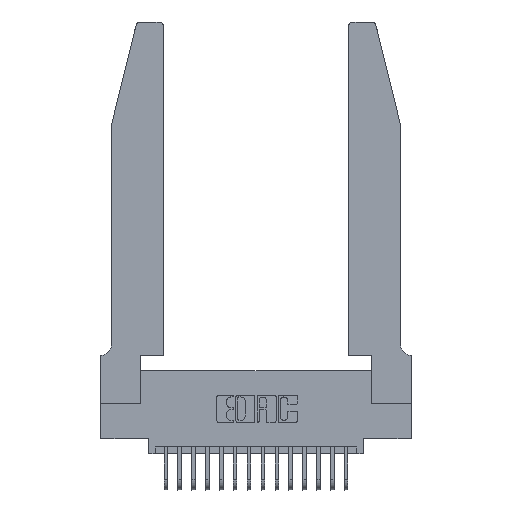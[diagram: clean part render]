
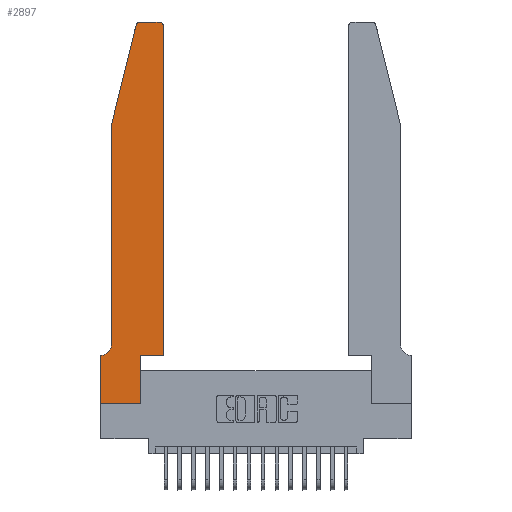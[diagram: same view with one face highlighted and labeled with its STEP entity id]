
A CAD part, top view. The second image highlights one B-rep face of the part: STEP entity #2897.
In plain terms, the highlighted planar face has unit normal (0, 0, 1).
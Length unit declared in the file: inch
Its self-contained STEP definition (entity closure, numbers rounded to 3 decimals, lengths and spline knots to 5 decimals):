
#325 = DIRECTION ( 'NONE',  ( -0.239, -0.971, 0. ) ) ;
#624 = DIRECTION ( 'NONE',  ( 0., 1., 0. ) ) ;
#640 = DIRECTION ( 'NONE',  ( 1., 0., 0. ) ) ;
#655 = VECTOR ( 'NONE', #14205, 39.37008 ) ;
#706 = EDGE_CURVE ( 'NONE', #8386, #5808, #14418, .T. ) ;
#888 = DIRECTION ( 'NONE',  ( 0., 0., 1. ) ) ;
#903 = ORIENTED_EDGE ( 'NONE', *, *, #10940, .T. ) ;
#1069 = LINE ( 'NONE', #20394, #10532 ) ;
#1198 = VERTEX_POINT ( 'NONE', #11049 ) ;
#1273 = DIRECTION ( 'NONE',  ( 0., 0., 1. ) ) ;
#1739 = DIRECTION ( 'NONE',  ( 0., 0., -1. ) ) ;
#1760 = VECTOR ( 'NONE', #624, 39.37008 ) ;
#2020 = CARTESIAN_POINT ( 'NONE',  ( 0.0755, 2., 0.37 ) ) ;
#2358 = VERTEX_POINT ( 'NONE', #17451 ) ;
#2367 = DIRECTION ( 'NONE',  ( 1., 0., 0. ) ) ;
#2600 = CARTESIAN_POINT ( 'NONE',  ( 0.4505, 0.35, 0.37 ) ) ;
#2601 = VECTOR ( 'NONE', #11731, 39.37008 ) ;
#2897 = ADVANCED_FACE ( 'NONE', ( #16101 ), #9296, .T. ) ;
#2921 = CARTESIAN_POINT ( 'NONE',  ( 0.284, 2.72, 0.37 ) ) ;
#3014 = CARTESIAN_POINT ( 'NONE',  ( 0.2865, 0.35, 0.37 ) ) ;
#3287 = CARTESIAN_POINT ( 'NONE',  ( 0.0755, 0.42, 0.37 ) ) ;
#3409 = CARTESIAN_POINT ( 'NONE',  ( 0.4205, 2.72, 0.37 ) ) ;
#3620 = VERTEX_POINT ( 'NONE', #20983 ) ;
#3639 = ORIENTED_EDGE ( 'NONE', *, *, #14645, .T. ) ;
#3955 = CARTESIAN_POINT ( 'NONE',  ( 0., 0., 0.37 ) ) ;
#4011 = EDGE_CURVE ( 'NONE', #3620, #1198, #1069, .T. ) ;
#4098 = ORIENTED_EDGE ( 'NONE', *, *, #18431, .T. ) ;
#4286 = EDGE_CURVE ( 'NONE', #17471, #16448, #14063, .T. ) ;
#4287 = CARTESIAN_POINT ( 'NONE',  ( 0.2865, 0., 0.37 ) ) ;
#4848 = VERTEX_POINT ( 'NONE', #5759 ) ;
#4916 = VECTOR ( 'NONE', #325, 39.37008 ) ;
#5116 = VERTEX_POINT ( 'NONE', #19408 ) ;
#5130 = DIRECTION ( 'NONE',  ( 1., 0., 0. ) ) ;
#5552 = LINE ( 'NONE', #20223, #8934 ) ;
#5682 = CARTESIAN_POINT ( 'NONE',  ( 0.2865, 0.35, 0.37 ) ) ;
#5715 = CARTESIAN_POINT ( 'NONE',  ( 0., 0., 0.37 ) ) ;
#5719 = AXIS2_PLACEMENT_3D ( 'NONE', #11769, #1739, #13392 ) ;
#5759 = CARTESIAN_POINT ( 'NONE',  ( 0.0755, 2., 0.37 ) ) ;
#5808 = VERTEX_POINT ( 'NONE', #10222 ) ;
#6016 = CARTESIAN_POINT ( 'NONE',  ( 0.284, 2.75, 0.37 ) ) ;
#6840 = ORIENTED_EDGE ( 'NONE', *, *, #20346, .T. ) ;
#6844 = LINE ( 'NONE', #5682, #1760 ) ;
#7094 = ORIENTED_EDGE ( 'NONE', *, *, #13338, .T. ) ;
#7664 = LINE ( 'NONE', #10010, #11496 ) ;
#8027 = EDGE_CURVE ( 'NONE', #1198, #17471, #7664, .T. ) ;
#8053 = EDGE_CURVE ( 'NONE', #4848, #12316, #15793, .T. ) ;
#8172 = DIRECTION ( 'NONE',  ( -1., 0., 0. ) ) ;
#8386 = VERTEX_POINT ( 'NONE', #6016 ) ;
#8934 = VECTOR ( 'NONE', #12210, 39.37008 ) ;
#9163 = AXIS2_PLACEMENT_3D ( 'NONE', #2921, #1273, #640 ) ;
#9296 = PLANE ( 'NONE',  #20408 ) ;
#9751 = VECTOR ( 'NONE', #2367, 39.37008 ) ;
#9823 = CARTESIAN_POINT ( 'NONE',  ( 0.2605, 2.75, 0.37 ) ) ;
#9972 = AXIS2_PLACEMENT_3D ( 'NONE', #3409, #14983, #5130 ) ;
#10010 = CARTESIAN_POINT ( 'NONE',  ( 0., 0., 0.37 ) ) ;
#10222 = CARTESIAN_POINT ( 'NONE',  ( 0.25487, 2.72718, 0.37 ) ) ;
#10316 = CIRCLE ( 'NONE', #9972, 0.03 ) ;
#10532 = VECTOR ( 'NONE', #10762, 39.37008 ) ;
#10707 = EDGE_CURVE ( 'NONE', #5808, #4848, #18473, .T. ) ;
#10762 = DIRECTION ( 'NONE',  ( -1., 0., 0. ) ) ;
#10932 = ORIENTED_EDGE ( 'NONE', *, *, #4011, .T. ) ;
#10940 = EDGE_CURVE ( 'NONE', #5116, #2358, #18214, .T. ) ;
#11049 = CARTESIAN_POINT ( 'NONE',  ( 0., 0.35, 0.37 ) ) ;
#11214 = EDGE_LOOP ( 'NONE', ( #7094, #18910, #15141, #12301, #3639, #10932, #19418, #18997, #16078, #6840, #903, #4098 ) ) ;
#11265 = VECTOR ( 'NONE', #8172, 39.37008 ) ;
#11496 = VECTOR ( 'NONE', #21220, 39.37008 ) ;
#11731 = DIRECTION ( 'NONE',  ( 0., -1., 0. ) ) ;
#11769 = CARTESIAN_POINT ( 'NONE',  ( 0.0055, 0.42, 0.37 ) ) ;
#12210 = DIRECTION ( 'NONE',  ( 1., 0., 0. ) ) ;
#12301 = ORIENTED_EDGE ( 'NONE', *, *, #8053, .T. ) ;
#12316 = VERTEX_POINT ( 'NONE', #3287 ) ;
#12563 = DIRECTION ( 'NONE',  ( 1., 0., 0. ) ) ;
#13246 = CIRCLE ( 'NONE', #5719, 0.07 ) ;
#13338 = EDGE_CURVE ( 'NONE', #13409, #8386, #19327, .T. ) ;
#13392 = DIRECTION ( 'NONE',  ( -1., 0., 0. ) ) ;
#13409 = VERTEX_POINT ( 'NONE', #16481 ) ;
#14063 = LINE ( 'NONE', #5715, #9751 ) ;
#14205 = DIRECTION ( 'NONE',  ( 0., 1., 0. ) ) ;
#14418 = CIRCLE ( 'NONE', #9163, 0.03 ) ;
#14505 = VERTEX_POINT ( 'NONE', #3014 ) ;
#14645 = EDGE_CURVE ( 'NONE', #12316, #3620, #13246, .T. ) ;
#14776 = EDGE_CURVE ( 'NONE', #16448, #14505, #6844, .T. ) ;
#14983 = DIRECTION ( 'NONE',  ( 0., 0., 1. ) ) ;
#15141 = ORIENTED_EDGE ( 'NONE', *, *, #10707, .T. ) ;
#15793 = LINE ( 'NONE', #18136, #2601 ) ;
#16078 = ORIENTED_EDGE ( 'NONE', *, *, #14776, .T. ) ;
#16101 = FACE_OUTER_BOUND ( 'NONE', #11214, .T. ) ;
#16448 = VERTEX_POINT ( 'NONE', #4287 ) ;
#16481 = CARTESIAN_POINT ( 'NONE',  ( 0.4205, 2.75, 0.37 ) ) ;
#17451 = CARTESIAN_POINT ( 'NONE',  ( 0.4505, 2.72, 0.37 ) ) ;
#17471 = VERTEX_POINT ( 'NONE', #3955 ) ;
#18136 = CARTESIAN_POINT ( 'NONE',  ( 0.0755, 2., 0.37 ) ) ;
#18214 = LINE ( 'NONE', #2600, #655 ) ;
#18431 = EDGE_CURVE ( 'NONE', #2358, #13409, #10316, .T. ) ;
#18473 = LINE ( 'NONE', #2020, #4916 ) ;
#18910 = ORIENTED_EDGE ( 'NONE', *, *, #706, .T. ) ;
#18997 = ORIENTED_EDGE ( 'NONE', *, *, #4286, .T. ) ;
#19327 = LINE ( 'NONE', #9823, #11265 ) ;
#19408 = CARTESIAN_POINT ( 'NONE',  ( 0.4505, 0.35, 0.37 ) ) ;
#19418 = ORIENTED_EDGE ( 'NONE', *, *, #8027, .T. ) ;
#20223 = CARTESIAN_POINT ( 'NONE',  ( 0.4505, 0.35, 0.37 ) ) ;
#20346 = EDGE_CURVE ( 'NONE', #14505, #5116, #5552, .T. ) ;
#20394 = CARTESIAN_POINT ( 'NONE',  ( 0.0755, 0.35, 0.37 ) ) ;
#20408 = AXIS2_PLACEMENT_3D ( 'NONE', #20582, #888, #12563 ) ;
#20582 = CARTESIAN_POINT ( 'NONE',  ( 0., 0.35, 0.37 ) ) ;
#20983 = CARTESIAN_POINT ( 'NONE',  ( 0.0055, 0.35, 0.37 ) ) ;
#21220 = DIRECTION ( 'NONE',  ( 0., -1., 0. ) ) ;
